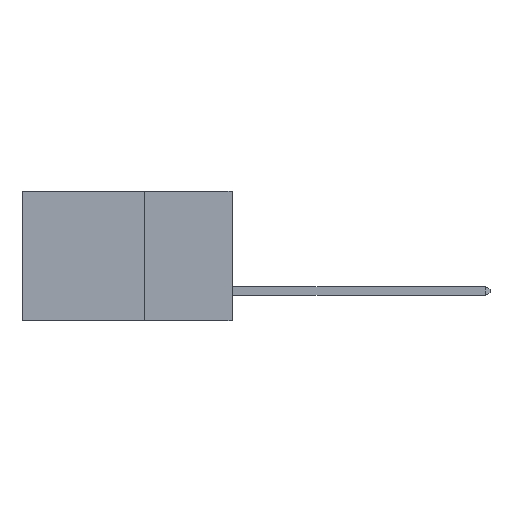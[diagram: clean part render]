
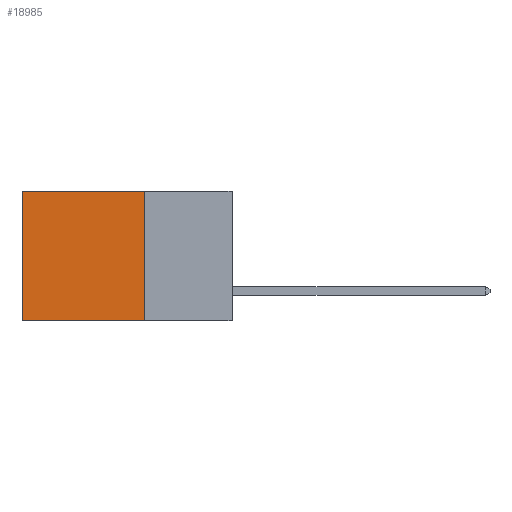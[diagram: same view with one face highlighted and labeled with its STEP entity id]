
A CAD part, left-side view. The second image highlights one B-rep face of the part: STEP entity #18985.
In plain terms, the highlighted planar face has unit normal (-1, 0, 0).
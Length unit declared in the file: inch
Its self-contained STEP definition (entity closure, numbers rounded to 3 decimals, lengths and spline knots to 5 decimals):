
#945 = EDGE_CURVE ( 'NONE', #10810, #21694, #22013, .T. ) ;
#1526 = DIRECTION ( 'NONE',  ( 0., 1., 0. ) ) ;
#1735 = CARTESIAN_POINT ( 'NONE',  ( 0.2875, 0.25, 0. ) ) ;
#2795 = CARTESIAN_POINT ( 'NONE',  ( 0.2875, 0.25, 0. ) ) ;
#3336 = DIRECTION ( 'NONE',  ( 1., 0., 0. ) ) ;
#3818 = CARTESIAN_POINT ( 'NONE',  ( 0.2875, 0.6, -0.37 ) ) ;
#4776 = ORIENTED_EDGE ( 'NONE', *, *, #18331, .T. ) ;
#4792 = ORIENTED_EDGE ( 'NONE', *, *, #11357, .T. ) ;
#4986 = FACE_OUTER_BOUND ( 'NONE', #19218, .T. ) ;
#5315 = LINE ( 'NONE', #2795, #20513 ) ;
#6426 = AXIS2_PLACEMENT_3D ( 'NONE', #7304, #3336, #16803 ) ;
#7304 = CARTESIAN_POINT ( 'NONE',  ( 0.2875, 0.25, 0. ) ) ;
#9359 = LINE ( 'NONE', #22519, #23684 ) ;
#9516 = CARTESIAN_POINT ( 'NONE',  ( 0.2875, 0.25, -0.37 ) ) ;
#10810 = VERTEX_POINT ( 'NONE', #24136 ) ;
#11323 = DIRECTION ( 'NONE',  ( 0., 0., -1. ) ) ;
#11357 = EDGE_CURVE ( 'NONE', #10810, #13411, #5315, .T. ) ;
#11631 = DIRECTION ( 'NONE',  ( 0., 0., -1. ) ) ;
#12510 = CARTESIAN_POINT ( 'NONE',  ( 0.2875, 0.25, -0.37 ) ) ;
#12781 = VERTEX_POINT ( 'NONE', #3818 ) ;
#13365 = ORIENTED_EDGE ( 'NONE', *, *, #945, .F. ) ;
#13411 = VERTEX_POINT ( 'NONE', #22068 ) ;
#16416 = ORIENTED_EDGE ( 'NONE', *, *, #21929, .F. ) ;
#16803 = DIRECTION ( 'NONE',  ( 0., 0., -1. ) ) ;
#17012 = VECTOR ( 'NONE', #11631, 39.37008 ) ;
#18222 = DIRECTION ( 'NONE',  ( 0., 1., 0. ) ) ;
#18272 = LINE ( 'NONE', #9516, #23223 ) ;
#18331 = EDGE_CURVE ( 'NONE', #13411, #12781, #9359, .T. ) ;
#18985 = ADVANCED_FACE ( 'NONE', ( #4986 ), #20457, .F. ) ;
#19218 = EDGE_LOOP ( 'NONE', ( #4776, #16416, #13365, #4792 ) ) ;
#20457 = PLANE ( 'NONE',  #6426 ) ;
#20513 = VECTOR ( 'NONE', #18222, 39.37008 ) ;
#21694 = VERTEX_POINT ( 'NONE', #12510 ) ;
#21929 = EDGE_CURVE ( 'NONE', #21694, #12781, #18272, .T. ) ;
#22013 = LINE ( 'NONE', #1735, #17012 ) ;
#22068 = CARTESIAN_POINT ( 'NONE',  ( 0.2875, 0.6, 0. ) ) ;
#22519 = CARTESIAN_POINT ( 'NONE',  ( 0.2875, 0.6, 0. ) ) ;
#23223 = VECTOR ( 'NONE', #1526, 39.37008 ) ;
#23684 = VECTOR ( 'NONE', #11323, 39.37008 ) ;
#24136 = CARTESIAN_POINT ( 'NONE',  ( 0.2875, 0.25, 0. ) ) ;
